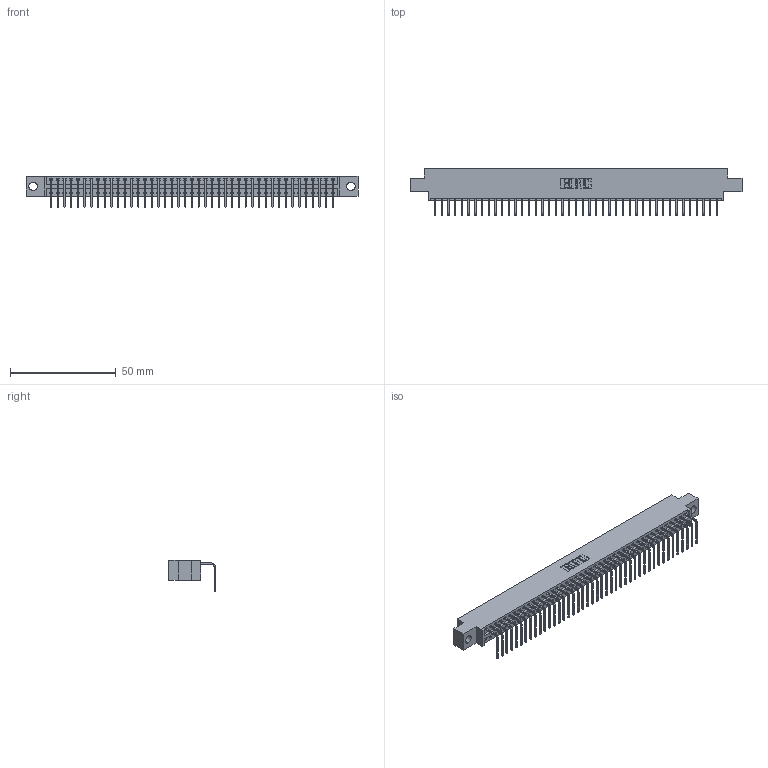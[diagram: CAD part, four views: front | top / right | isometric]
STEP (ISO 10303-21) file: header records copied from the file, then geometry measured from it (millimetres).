
FILE_DESCRIPTION (( 'STEP AP203' ), '1' );
FILE_NAME ('346-043-558-604.STEP', '2022-05-09T16:13:01', ( '' ), ( '' ), 'SwSTEP 2.0', 'SolidWorks 2020', '' );
FILE_SCHEMA (( 'CONFIG_CONTROL_DESIGN' ));
Length unit declared in the file: inch
Products named in the file (3): 346 Part_0.170 Offset - 0.156 Dia-TH; 345-292-001_558 Tail - 2; 346-043-558-604
Assembly tree (44 placements, depth 2):
  346-043-558-604
    346 Part_0.170 Offset - 0.156 Dia-TH
    345-292-001_558 Tail - 2  x43
Bounding box: 157.1 x 22.16 x 14.73 mm (x, y, z)
Volume: 14927.4 mm3; surface area: 19520.5 mm2
Topology: 44 solids, 44 shells, 2720 faces, 8203 edges, 5410 vertices
Faces by surface type: plane 1900, cylinder 820
Entity records: 27187 total; most frequent: CARTESIAN_POINT 4671, ORIENTED_EDGE 4646, DIRECTION 4117, EDGE_CURVE 2323, VECTOR 2019, LINE 2019, VERTEX_POINT 1546, AXIS2_PLACEMENT_3D 1049
